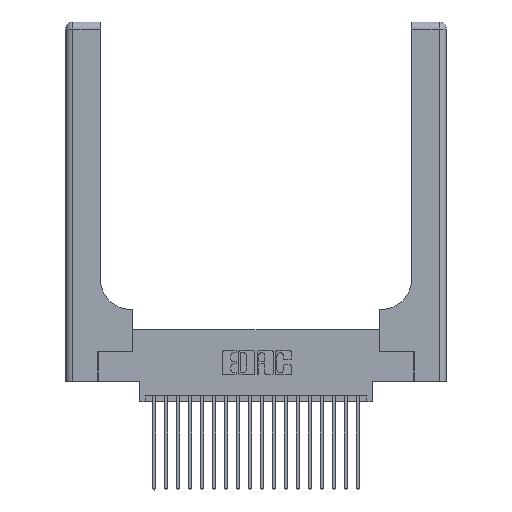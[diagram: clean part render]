
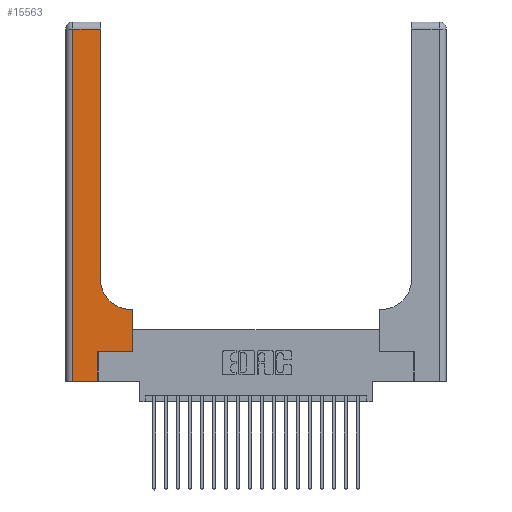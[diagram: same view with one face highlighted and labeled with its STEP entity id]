
A CAD part, top view. The second image highlights one B-rep face of the part: STEP entity #15563.
In plain terms, the highlighted planar face has unit normal (0, 0, 1).
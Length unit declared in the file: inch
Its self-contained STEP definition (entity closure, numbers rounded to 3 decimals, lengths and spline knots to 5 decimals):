
#516 = VERTEX_POINT ( 'NONE', #7212 ) ;
#527 = VERTEX_POINT ( 'NONE', #14114 ) ;
#534 = VECTOR ( 'NONE', #15816, 39.37008 ) ;
#1423 = CARTESIAN_POINT ( 'NONE',  ( 0., 3., 0.37 ) ) ;
#1817 = VERTEX_POINT ( 'NONE', #6258 ) ;
#2256 = LINE ( 'NONE', #13853, #17380 ) ;
#3239 = VERTEX_POINT ( 'NONE', #6480 ) ;
#3581 = VERTEX_POINT ( 'NONE', #10973 ) ;
#3859 = ORIENTED_EDGE ( 'NONE', *, *, #17265, .T. ) ;
#4191 = VECTOR ( 'NONE', #13705, 39.37008 ) ;
#4634 = DIRECTION ( 'NONE',  ( -1., 0., 0. ) ) ;
#4892 = CARTESIAN_POINT ( 'NONE',  ( 0.5585, 0.6, 0.37 ) ) ;
#5284 = AXIS2_PLACEMENT_3D ( 'NONE', #1423, #22401, #9984 ) ;
#5715 = ORIENTED_EDGE ( 'NONE', *, *, #7652, .T. ) ;
#6220 = VECTOR ( 'NONE', #16441, 39.37008 ) ;
#6258 = CARTESIAN_POINT ( 'NONE',  ( 0.06, 0., 0.37 ) ) ;
#6448 = VECTOR ( 'NONE', #10169, 39.37008 ) ;
#6480 = CARTESIAN_POINT ( 'NONE',  ( 0.269, 0.25, 0.37 ) ) ;
#6586 = LINE ( 'NONE', #13326, #16399 ) ;
#6816 = CARTESIAN_POINT ( 'NONE',  ( 0., 2.94, 0.37 ) ) ;
#6871 = VERTEX_POINT ( 'NONE', #10070 ) ;
#7212 = CARTESIAN_POINT ( 'NONE',  ( 0.06, 2.94, 0.37 ) ) ;
#7403 = CARTESIAN_POINT ( 'NONE',  ( 0.5415, 0.85, 0.37 ) ) ;
#7652 = EDGE_CURVE ( 'NONE', #20245, #527, #6586, .T. ) ;
#8312 = DIRECTION ( 'NONE',  ( 0., 1., 0. ) ) ;
#8337 = AXIS2_PLACEMENT_3D ( 'NONE', #7403, #10883, #9318 ) ;
#8459 = CARTESIAN_POINT ( 'NONE',  ( 0.06, 3., 0.37 ) ) ;
#8699 = CARTESIAN_POINT ( 'NONE',  ( 0.5585, 0.25, 0.37 ) ) ;
#9318 = DIRECTION ( 'NONE',  ( 1., 0., 0. ) ) ;
#9383 = DIRECTION ( 'NONE',  ( 0., 1., 0. ) ) ;
#9720 = ORIENTED_EDGE ( 'NONE', *, *, #17263, .T. ) ;
#9790 = LINE ( 'NONE', #21638, #6220 ) ;
#9984 = DIRECTION ( 'NONE',  ( -1., 0., 0. ) ) ;
#10070 = CARTESIAN_POINT ( 'NONE',  ( 0.5585, 0.25, 0.37 ) ) ;
#10169 = DIRECTION ( 'NONE',  ( 0., -1., 0. ) ) ;
#10699 = EDGE_CURVE ( 'NONE', #1817, #18862, #9790, .T. ) ;
#10883 = DIRECTION ( 'NONE',  ( 0., 0., -1. ) ) ;
#10973 = CARTESIAN_POINT ( 'NONE',  ( 0.2915, 2.94, 0.37 ) ) ;
#11033 = LINE ( 'NONE', #6816, #534 ) ;
#11509 = ORIENTED_EDGE ( 'NONE', *, *, #19233, .T. ) ;
#12831 = CARTESIAN_POINT ( 'NONE',  ( 0.269, 0., 0.37 ) ) ;
#13326 = CARTESIAN_POINT ( 'NONE',  ( 0.2915, 0.6, 0.37 ) ) ;
#13349 = EDGE_CURVE ( 'NONE', #18862, #3239, #19800, .T. ) ;
#13587 = ORIENTED_EDGE ( 'NONE', *, *, #21346, .T. ) ;
#13705 = DIRECTION ( 'NONE',  ( 0., 1., 0. ) ) ;
#13853 = CARTESIAN_POINT ( 'NONE',  ( 0.2915, 3., 0.37 ) ) ;
#14114 = CARTESIAN_POINT ( 'NONE',  ( 0.5415, 0.6, 0.37 ) ) ;
#14366 = LINE ( 'NONE', #8459, #6448 ) ;
#14609 = EDGE_CURVE ( 'NONE', #527, #16335, #14823, .T. ) ;
#14823 = CIRCLE ( 'NONE', #8337, 0.25 ) ;
#15006 = CARTESIAN_POINT ( 'NONE',  ( 0.269, 0.25, 0.37 ) ) ;
#15322 = FACE_OUTER_BOUND ( 'NONE', #16700, .T. ) ;
#15563 = ADVANCED_FACE ( 'NONE', ( #15322 ), #20436, .F. ) ;
#15809 = ORIENTED_EDGE ( 'NONE', *, *, #10699, .T. ) ;
#15816 = DIRECTION ( 'NONE',  ( -1., 0., 0. ) ) ;
#16335 = VERTEX_POINT ( 'NONE', #17452 ) ;
#16399 = VECTOR ( 'NONE', #4634, 39.37008 ) ;
#16441 = DIRECTION ( 'NONE',  ( 1., 0., 0. ) ) ;
#16700 = EDGE_LOOP ( 'NONE', ( #17779, #11509, #3859, #15809, #17784, #13587, #9720, #5715, #19027 ) ) ;
#17156 = EDGE_CURVE ( 'NONE', #16335, #3581, #2256, .T. ) ;
#17263 = EDGE_CURVE ( 'NONE', #6871, #20245, #20883, .T. ) ;
#17265 = EDGE_CURVE ( 'NONE', #516, #1817, #14366, .T. ) ;
#17380 = VECTOR ( 'NONE', #8312, 39.37008 ) ;
#17452 = CARTESIAN_POINT ( 'NONE',  ( 0.2915, 0.85, 0.37 ) ) ;
#17779 = ORIENTED_EDGE ( 'NONE', *, *, #17156, .T. ) ;
#17784 = ORIENTED_EDGE ( 'NONE', *, *, #13349, .T. ) ;
#18691 = VECTOR ( 'NONE', #9383, 39.37008 ) ;
#18815 = LINE ( 'NONE', #15006, #20183 ) ;
#18862 = VERTEX_POINT ( 'NONE', #12831 ) ;
#19027 = ORIENTED_EDGE ( 'NONE', *, *, #14609, .T. ) ;
#19233 = EDGE_CURVE ( 'NONE', #3581, #516, #11033, .T. ) ;
#19800 = LINE ( 'NONE', #21430, #18691 ) ;
#19984 = DIRECTION ( 'NONE',  ( 1., 0., 0. ) ) ;
#20183 = VECTOR ( 'NONE', #19984, 39.37008 ) ;
#20245 = VERTEX_POINT ( 'NONE', #4892 ) ;
#20436 = PLANE ( 'NONE',  #5284 ) ;
#20883 = LINE ( 'NONE', #8699, #4191 ) ;
#21346 = EDGE_CURVE ( 'NONE', #3239, #6871, #18815, .T. ) ;
#21430 = CARTESIAN_POINT ( 'NONE',  ( 0.269, 0., 0.37 ) ) ;
#21638 = CARTESIAN_POINT ( 'NONE',  ( 0., 0., 0.37 ) ) ;
#22401 = DIRECTION ( 'NONE',  ( 0., 0., -1. ) ) ;
